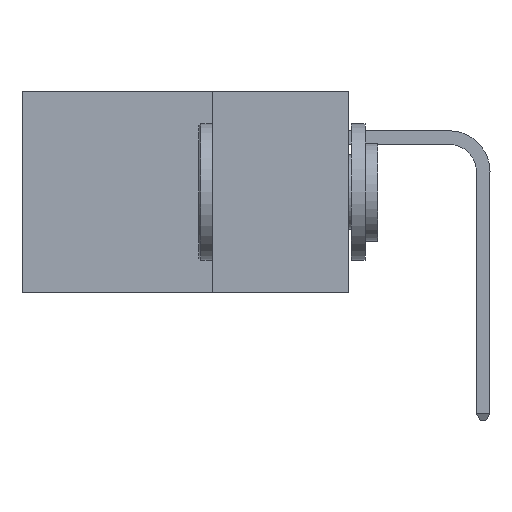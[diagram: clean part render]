
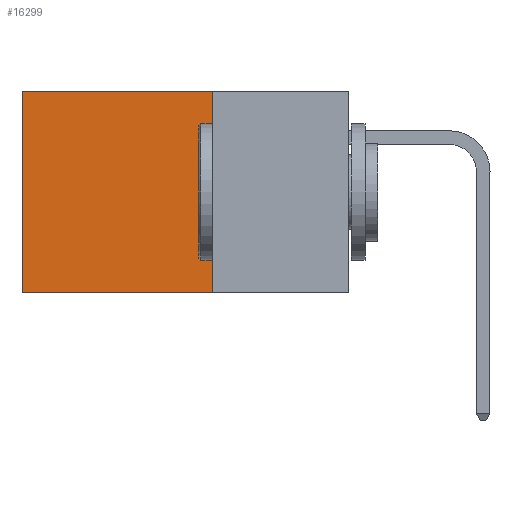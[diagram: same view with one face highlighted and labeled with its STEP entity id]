
A CAD part, left-side view. The second image highlights one B-rep face of the part: STEP entity #16299.
In plain terms, the highlighted planar face has unit normal (-1, 0, 0).
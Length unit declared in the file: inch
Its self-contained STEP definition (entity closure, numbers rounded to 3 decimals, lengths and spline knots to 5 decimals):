
#313 = CARTESIAN_POINT ( 'NONE',  ( 0.2875, 0.25, -0.37 ) ) ;
#640 = CARTESIAN_POINT ( 'NONE',  ( 0.2875, 0.6, 0. ) ) ;
#808 = VECTOR ( 'NONE', #1674, 39.37008 ) ;
#1674 = DIRECTION ( 'NONE',  ( 0., 1., 0. ) ) ;
#2610 = VERTEX_POINT ( 'NONE', #13804 ) ;
#2910 = CARTESIAN_POINT ( 'NONE',  ( 0.2875, 0.25, 0. ) ) ;
#3584 = DIRECTION ( 'NONE',  ( 0., 1., 0. ) ) ;
#3666 = VECTOR ( 'NONE', #3584, 39.37008 ) ;
#3683 = EDGE_CURVE ( 'NONE', #2610, #7489, #16275, .T. ) ;
#3854 = LINE ( 'NONE', #18572, #11083 ) ;
#3903 = LINE ( 'NONE', #7765, #808 ) ;
#4906 = ORIENTED_EDGE ( 'NONE', *, *, #3683, .T. ) ;
#5486 = DIRECTION ( 'NONE',  ( 0., 0., -1. ) ) ;
#5518 = AXIS2_PLACEMENT_3D ( 'NONE', #2910, #17863, #17924 ) ;
#7194 = LINE ( 'NONE', #14416, #18654 ) ;
#7489 = VERTEX_POINT ( 'NONE', #640 ) ;
#7765 = CARTESIAN_POINT ( 'NONE',  ( 0.2875, 0.25, -0.37 ) ) ;
#7919 = EDGE_LOOP ( 'NONE', ( #9752, #14591, #11022, #4906 ) ) ;
#8442 = EDGE_CURVE ( 'NONE', #7489, #16463, #7194, .T. ) ;
#9594 = DIRECTION ( 'NONE',  ( 0., 0., -1. ) ) ;
#9706 = FACE_OUTER_BOUND ( 'NONE', #7919, .T. ) ;
#9752 = ORIENTED_EDGE ( 'NONE', *, *, #8442, .T. ) ;
#10771 = EDGE_CURVE ( 'NONE', #17633, #16463, #3903, .T. ) ;
#11022 = ORIENTED_EDGE ( 'NONE', *, *, #11643, .F. ) ;
#11083 = VECTOR ( 'NONE', #9594, 39.37008 ) ;
#11643 = EDGE_CURVE ( 'NONE', #2610, #17633, #3854, .T. ) ;
#13804 = CARTESIAN_POINT ( 'NONE',  ( 0.2875, 0.25, 0. ) ) ;
#14416 = CARTESIAN_POINT ( 'NONE',  ( 0.2875, 0.6, 0. ) ) ;
#14591 = ORIENTED_EDGE ( 'NONE', *, *, #10771, .F. ) ;
#16275 = LINE ( 'NONE', #16769, #3666 ) ;
#16299 = ADVANCED_FACE ( 'NONE', ( #9706 ), #16305, .F. ) ;
#16305 = PLANE ( 'NONE',  #5518 ) ;
#16463 = VERTEX_POINT ( 'NONE', #17065 ) ;
#16769 = CARTESIAN_POINT ( 'NONE',  ( 0.2875, 0.25, 0. ) ) ;
#17065 = CARTESIAN_POINT ( 'NONE',  ( 0.2875, 0.6, -0.37 ) ) ;
#17633 = VERTEX_POINT ( 'NONE', #313 ) ;
#17863 = DIRECTION ( 'NONE',  ( 1., 0., 0. ) ) ;
#17924 = DIRECTION ( 'NONE',  ( 0., 0., -1. ) ) ;
#18572 = CARTESIAN_POINT ( 'NONE',  ( 0.2875, 0.25, 0. ) ) ;
#18654 = VECTOR ( 'NONE', #5486, 39.37008 ) ;
